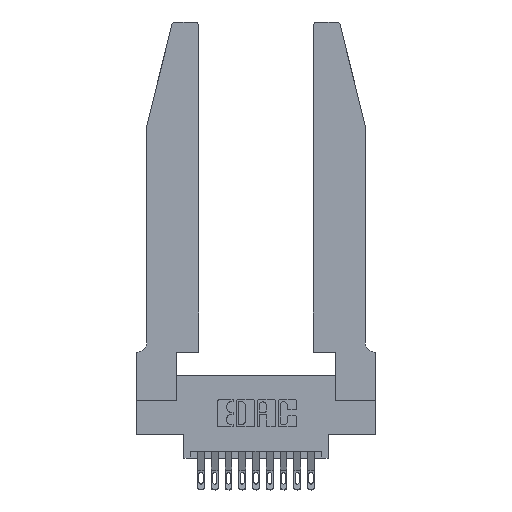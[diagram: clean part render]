
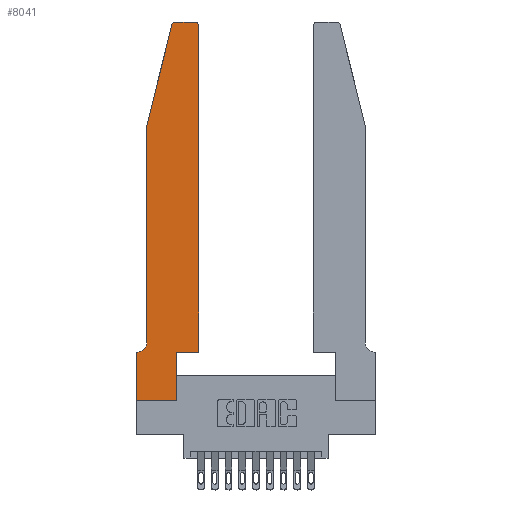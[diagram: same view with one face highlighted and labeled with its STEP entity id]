
A CAD part, top view. The second image highlights one B-rep face of the part: STEP entity #8041.
In plain terms, the highlighted planar face has unit normal (0, 0, 1).
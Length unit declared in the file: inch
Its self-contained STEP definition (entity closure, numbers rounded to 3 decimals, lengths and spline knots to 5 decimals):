
#311 = ORIENTED_EDGE ( 'NONE', *, *, #6223, .T. ) ;
#514 = CARTESIAN_POINT ( 'NONE',  ( 0.0755, 2., 0.37 ) ) ;
#749 = VERTEX_POINT ( 'NONE', #9967 ) ;
#802 = AXIS2_PLACEMENT_3D ( 'NONE', #8393, #7017, #4339 ) ;
#965 = EDGE_CURVE ( 'NONE', #10162, #14302, #14226, .T. ) ;
#1170 = CARTESIAN_POINT ( 'NONE',  ( 0.0755, 0.42, 0.37 ) ) ;
#1174 = LINE ( 'NONE', #514, #4177 ) ;
#1352 = AXIS2_PLACEMENT_3D ( 'NONE', #6718, #7110, #9984 ) ;
#1538 = DIRECTION ( 'NONE',  ( 0., 0., 1. ) ) ;
#1560 = VERTEX_POINT ( 'NONE', #2651 ) ;
#1587 = CARTESIAN_POINT ( 'NONE',  ( 0.0755, 2., 0.37 ) ) ;
#1785 = DIRECTION ( 'NONE',  ( 0., -1., 0. ) ) ;
#2025 = FACE_OUTER_BOUND ( 'NONE', #12088, .T. ) ;
#2619 = DIRECTION ( 'NONE',  ( -0.239, -0.971, 0. ) ) ;
#2651 = CARTESIAN_POINT ( 'NONE',  ( 0.0755, 2., 0.37 ) ) ;
#2690 = EDGE_CURVE ( 'NONE', #749, #6140, #10944, .T. ) ;
#3099 = CARTESIAN_POINT ( 'NONE',  ( 0.0755, 0.35, 0.37 ) ) ;
#3160 = VERTEX_POINT ( 'NONE', #4626 ) ;
#3355 = ORIENTED_EDGE ( 'NONE', *, *, #3737, .T. ) ;
#3394 = DIRECTION ( 'NONE',  ( 1., 0., 0. ) ) ;
#3455 = CARTESIAN_POINT ( 'NONE',  ( 0.4505, 0.35, 0.37 ) ) ;
#3557 = ORIENTED_EDGE ( 'NONE', *, *, #965, .T. ) ;
#3663 = EDGE_CURVE ( 'NONE', #5948, #3160, #16478, .T. ) ;
#3737 = EDGE_CURVE ( 'NONE', #15092, #8702, #13056, .T. ) ;
#3866 = ORIENTED_EDGE ( 'NONE', *, *, #9380, .T. ) ;
#3938 = DIRECTION ( 'NONE',  ( 1., 0., 0. ) ) ;
#3988 = CARTESIAN_POINT ( 'NONE',  ( 0., 0., 0.37 ) ) ;
#4147 = CARTESIAN_POINT ( 'NONE',  ( 0., 0., 0.37 ) ) ;
#4177 = VECTOR ( 'NONE', #1785, 39.37008 ) ;
#4339 = DIRECTION ( 'NONE',  ( 1., 0., 0. ) ) ;
#4626 = CARTESIAN_POINT ( 'NONE',  ( 0.25487, 2.72718, 0.37 ) ) ;
#5018 = ORIENTED_EDGE ( 'NONE', *, *, #5351, .T. ) ;
#5142 = DIRECTION ( 'NONE',  ( 1., 0., 0. ) ) ;
#5326 = VECTOR ( 'NONE', #12501, 39.37008 ) ;
#5351 = EDGE_CURVE ( 'NONE', #8702, #5948, #8965, .T. ) ;
#5438 = VERTEX_POINT ( 'NONE', #7168 ) ;
#5818 = PLANE ( 'NONE',  #802 ) ;
#5898 = VECTOR ( 'NONE', #2619, 39.37008 ) ;
#5948 = VERTEX_POINT ( 'NONE', #7579 ) ;
#6049 = LINE ( 'NONE', #8463, #11093 ) ;
#6140 = VERTEX_POINT ( 'NONE', #3988 ) ;
#6214 = ORIENTED_EDGE ( 'NONE', *, *, #2690, .T. ) ;
#6223 = EDGE_CURVE ( 'NONE', #14302, #749, #16607, .T. ) ;
#6718 = CARTESIAN_POINT ( 'NONE',  ( 0.0055, 0.42, 0.37 ) ) ;
#7017 = DIRECTION ( 'NONE',  ( 0., 0., 1. ) ) ;
#7110 = DIRECTION ( 'NONE',  ( 0., 0., -1. ) ) ;
#7168 = CARTESIAN_POINT ( 'NONE',  ( 0.2865, 0.35, 0.37 ) ) ;
#7290 = LINE ( 'NONE', #13734, #10133 ) ;
#7579 = CARTESIAN_POINT ( 'NONE',  ( 0.284, 2.75, 0.37 ) ) ;
#7627 = LINE ( 'NONE', #16667, #8047 ) ;
#7664 = AXIS2_PLACEMENT_3D ( 'NONE', #8320, #1538, #3938 ) ;
#7932 = VECTOR ( 'NONE', #9550, 39.37008 ) ;
#8041 = ADVANCED_FACE ( 'NONE', ( #2025 ), #5818, .T. ) ;
#8047 = VECTOR ( 'NONE', #16539, 39.37008 ) ;
#8174 = CARTESIAN_POINT ( 'NONE',  ( 0.2865, 0., 0.37 ) ) ;
#8320 = CARTESIAN_POINT ( 'NONE',  ( 0.284, 2.72, 0.37 ) ) ;
#8346 = ORIENTED_EDGE ( 'NONE', *, *, #14676, .T. ) ;
#8393 = CARTESIAN_POINT ( 'NONE',  ( 0., 0.35, 0.37 ) ) ;
#8463 = CARTESIAN_POINT ( 'NONE',  ( 0., 0., 0.37 ) ) ;
#8648 = ORIENTED_EDGE ( 'NONE', *, *, #8913, .T. ) ;
#8702 = VERTEX_POINT ( 'NONE', #10562 ) ;
#8913 = EDGE_CURVE ( 'NONE', #1560, #10162, #1174, .T. ) ;
#8965 = LINE ( 'NONE', #14918, #16419 ) ;
#9234 = LINE ( 'NONE', #3455, #5326 ) ;
#9380 = EDGE_CURVE ( 'NONE', #12637, #15092, #7627, .T. ) ;
#9550 = DIRECTION ( 'NONE',  ( -1., 0., 0. ) ) ;
#9967 = CARTESIAN_POINT ( 'NONE',  ( 0., 0.35, 0.37 ) ) ;
#9984 = DIRECTION ( 'NONE',  ( -1., 0., 0. ) ) ;
#10131 = ORIENTED_EDGE ( 'NONE', *, *, #15727, .T. ) ;
#10133 = VECTOR ( 'NONE', #15083, 39.37008 ) ;
#10162 = VERTEX_POINT ( 'NONE', #1170 ) ;
#10562 = CARTESIAN_POINT ( 'NONE',  ( 0.4205, 2.75, 0.37 ) ) ;
#10944 = LINE ( 'NONE', #4147, #16387 ) ;
#11021 = ORIENTED_EDGE ( 'NONE', *, *, #13557, .T. ) ;
#11093 = VECTOR ( 'NONE', #3394, 39.37008 ) ;
#11212 = VERTEX_POINT ( 'NONE', #8174 ) ;
#11367 = EDGE_CURVE ( 'NONE', #5438, #12637, #9234, .T. ) ;
#11781 = LINE ( 'NONE', #1587, #5898 ) ;
#11843 = CARTESIAN_POINT ( 'NONE',  ( 0.4205, 2.72, 0.37 ) ) ;
#12088 = EDGE_LOOP ( 'NONE', ( #5018, #14909, #11021, #8648, #3557, #311, #6214, #10131, #8346, #14946, #3866, #3355 ) ) ;
#12225 = CARTESIAN_POINT ( 'NONE',  ( 0.4505, 2.72, 0.37 ) ) ;
#12292 = AXIS2_PLACEMENT_3D ( 'NONE', #11843, #16525, #5142 ) ;
#12351 = CARTESIAN_POINT ( 'NONE',  ( 0.0055, 0.35, 0.37 ) ) ;
#12501 = DIRECTION ( 'NONE',  ( 1., 0., 0. ) ) ;
#12637 = VERTEX_POINT ( 'NONE', #16028 ) ;
#13056 = CIRCLE ( 'NONE', #12292, 0.03 ) ;
#13388 = DIRECTION ( 'NONE',  ( 0., -1., 0. ) ) ;
#13557 = EDGE_CURVE ( 'NONE', #3160, #1560, #11781, .T. ) ;
#13734 = CARTESIAN_POINT ( 'NONE',  ( 0.2865, 0.35, 0.37 ) ) ;
#14226 = CIRCLE ( 'NONE', #1352, 0.07 ) ;
#14302 = VERTEX_POINT ( 'NONE', #12351 ) ;
#14676 = EDGE_CURVE ( 'NONE', #11212, #5438, #7290, .T. ) ;
#14909 = ORIENTED_EDGE ( 'NONE', *, *, #3663, .T. ) ;
#14918 = CARTESIAN_POINT ( 'NONE',  ( 0.2605, 2.75, 0.37 ) ) ;
#14946 = ORIENTED_EDGE ( 'NONE', *, *, #11367, .T. ) ;
#15083 = DIRECTION ( 'NONE',  ( 0., 1., 0. ) ) ;
#15092 = VERTEX_POINT ( 'NONE', #12225 ) ;
#15727 = EDGE_CURVE ( 'NONE', #6140, #11212, #6049, .T. ) ;
#16028 = CARTESIAN_POINT ( 'NONE',  ( 0.4505, 0.35, 0.37 ) ) ;
#16082 = DIRECTION ( 'NONE',  ( -1., 0., 0. ) ) ;
#16387 = VECTOR ( 'NONE', #13388, 39.37008 ) ;
#16419 = VECTOR ( 'NONE', #16082, 39.37008 ) ;
#16478 = CIRCLE ( 'NONE', #7664, 0.03 ) ;
#16525 = DIRECTION ( 'NONE',  ( 0., 0., 1. ) ) ;
#16539 = DIRECTION ( 'NONE',  ( 0., 1., 0. ) ) ;
#16607 = LINE ( 'NONE', #3099, #7932 ) ;
#16667 = CARTESIAN_POINT ( 'NONE',  ( 0.4505, 0.35, 0.37 ) ) ;
